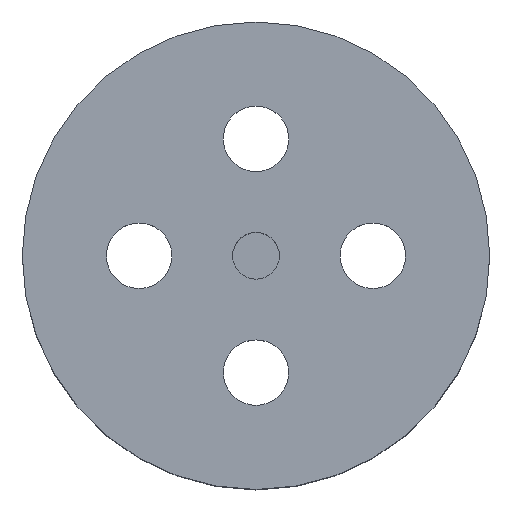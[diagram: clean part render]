
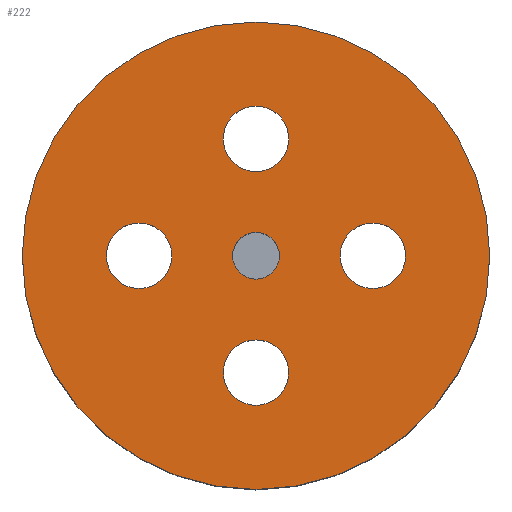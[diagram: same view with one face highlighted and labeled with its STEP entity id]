
A CAD part, top view. The second image highlights one B-rep face of the part: STEP entity #222.
In plain terms, the highlighted planar face has unit normal (0, 0, 1).
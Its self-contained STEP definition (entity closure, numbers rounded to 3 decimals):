
#18 = ORIENTED_EDGE ( 'NONE', *, *, #85, .F. ) ;
#62 = EDGE_CURVE ( 'NONE', #857, #853, #886, .T. ) ;
#64 = EDGE_CURVE ( 'NONE', #859, #860, #882, .T. ) ;
#68 = EDGE_CURVE ( 'NONE', #858, #1016, #864, .T. ) ;
#73 = EDGE_CURVE ( 'NONE', #861, #1049, #862, .T. ) ;
#85 = EDGE_CURVE ( 'NONE', #769, #775, #551, .T. ) ;
#86 = EDGE_CURVE ( 'NONE', #1076, #1083, #544, .T. ) ;
#87 = EDGE_CURVE ( 'NONE', #1049, #861, #519, .T. ) ;
#88 = EDGE_CURVE ( 'NONE', #1016, #858, #550, .T. ) ;
#89 = EDGE_CURVE ( 'NONE', #853, #857, #558, .T. ) ;
#90 = EDGE_CURVE ( 'NONE', #860, #859, #559, .T. ) ;
#101 = EDGE_CURVE ( 'NONE', #775, #769, #538, .T. ) ;
#116 = AXIS2_PLACEMENT_3D ( 'NONE', #666, #665, #660 ) ;
#117 = AXIS2_PLACEMENT_3D ( 'NONE', #662, #659, #658 ) ;
#120 = AXIS2_PLACEMENT_3D ( 'NONE', #636, #621, #619 ) ;
#122 = AXIS2_PLACEMENT_3D ( 'NONE', #591, #635, #608 ) ;
#128 = AXIS2_PLACEMENT_3D ( 'NONE', #626, #625, #598 ) ;
#129 = AXIS2_PLACEMENT_3D ( 'NONE', #642, #640, #639 ) ;
#130 = AXIS2_PLACEMENT_3D ( 'NONE', #652, #654, #628 ) ;
#131 = AXIS2_PLACEMENT_3D ( 'NONE', #651, #638, #627 ) ;
#132 = AXIS2_PLACEMENT_3D ( 'NONE', #630, #607, #606 ) ;
#133 = AXIS2_PLACEMENT_3D ( 'NONE', #1129, #1096, #1113 ) ;
#137 = AXIS2_PLACEMENT_3D ( 'NONE', #1097, #1091, #1127 ) ;
#155 = AXIS2_PLACEMENT_3D ( 'NONE', #252, #254, #255 ) ;
#184 = AXIS2_PLACEMENT_3D ( 'NONE', #392, #393, #394 ) ;
#222 = ADVANCED_FACE ( 'NONE', ( #529, #553, #557, #505, #562, #517 ), #251, .T. ) ;
#251 = PLANE ( 'NONE',  #155 ) ;
#252 = CARTESIAN_POINT ( 'NONE',  ( 0., 0., 30. ) ) ;
#254 = DIRECTION ( 'NONE',  ( 0., 0., 1. ) ) ;
#255 = DIRECTION ( 'NONE',  ( 1., 0., 0. ) ) ;
#352 = CARTESIAN_POINT ( 'NONE',  ( -3.5, 12.5, 30. ) ) ;
#357 = CARTESIAN_POINT ( 'NONE',  ( 2.5, 0., 30. ) ) ;
#358 = CARTESIAN_POINT ( 'NONE',  ( -2.5, 0., 30. ) ) ;
#364 = CARTESIAN_POINT ( 'NONE',  ( -16., 0., 30. ) ) ;
#365 = CARTESIAN_POINT ( 'NONE',  ( 3.5, -12.5, 30. ) ) ;
#367 = CARTESIAN_POINT ( 'NONE',  ( -3.5, -12.5, 30. ) ) ;
#368 = CARTESIAN_POINT ( 'NONE',  ( 9., 0., 30. ) ) ;
#369 = CARTESIAN_POINT ( 'NONE',  ( 16., 0., 30. ) ) ;
#392 = CARTESIAN_POINT ( 'NONE',  ( 0., 0., 30. ) ) ;
#393 = DIRECTION ( 'NONE',  ( 0., 0., 1. ) ) ;
#394 = DIRECTION ( 'NONE',  ( 1., 0., 0. ) ) ;
#396 = CARTESIAN_POINT ( 'NONE',  ( -9., 0., 30. ) ) ;
#422 = CARTESIAN_POINT ( 'NONE',  ( 3.5, 12.5, 30. ) ) ;
#428 = CARTESIAN_POINT ( 'NONE',  ( -25., 0., 30. ) ) ;
#440 = CARTESIAN_POINT ( 'NONE',  ( 25., 0., 30. ) ) ;
#505 = FACE_BOUND ( 'NONE', #1166, .T. ) ;
#517 = FACE_BOUND ( 'NONE', #1155, .T. ) ;
#519 = CIRCLE ( 'NONE', #130, 3.5 ) ;
#529 = FACE_BOUND ( 'NONE', #1050, .T. ) ;
#538 = CIRCLE ( 'NONE', #137, 2.5 ) ;
#544 = CIRCLE ( 'NONE', #129, 25. ) ;
#550 = CIRCLE ( 'NONE', #131, 3.5 ) ;
#551 = CIRCLE ( 'NONE', #128, 2.5 ) ;
#553 = FACE_BOUND ( 'NONE', #1216, .T. ) ;
#557 = FACE_BOUND ( 'NONE', #1028, .T. ) ;
#558 = CIRCLE ( 'NONE', #132, 3.5 ) ;
#559 = CIRCLE ( 'NONE', #133, 3.5 ) ;
#562 = FACE_OUTER_BOUND ( 'NONE', #1225, .T. ) ;
#591 = CARTESIAN_POINT ( 'NONE',  ( 0., 12.5, 30. ) ) ;
#598 = DIRECTION ( 'NONE',  ( 1., 0., 0. ) ) ;
#606 = DIRECTION ( 'NONE',  ( 1., 0., 0. ) ) ;
#607 = DIRECTION ( 'NONE',  ( 0., 0., 1. ) ) ;
#608 = DIRECTION ( 'NONE',  ( 1., 0., 0. ) ) ;
#619 = DIRECTION ( 'NONE',  ( 1., 0., 0. ) ) ;
#621 = DIRECTION ( 'NONE',  ( 0., 0., 1. ) ) ;
#625 = DIRECTION ( 'NONE',  ( 0., 0., 1. ) ) ;
#626 = CARTESIAN_POINT ( 'NONE',  ( 0., 0., 30. ) ) ;
#627 = DIRECTION ( 'NONE',  ( 1., 0., 0. ) ) ;
#628 = DIRECTION ( 'NONE',  ( 1., 0., 0. ) ) ;
#630 = CARTESIAN_POINT ( 'NONE',  ( 0., -12.5, 30. ) ) ;
#635 = DIRECTION ( 'NONE',  ( 0., 0., 1. ) ) ;
#636 = CARTESIAN_POINT ( 'NONE',  ( -12.5, 0., 30. ) ) ;
#638 = DIRECTION ( 'NONE',  ( 0., 0., 1. ) ) ;
#639 = DIRECTION ( 'NONE',  ( 1., 0., 0. ) ) ;
#640 = DIRECTION ( 'NONE',  ( 0., 0., 1. ) ) ;
#642 = CARTESIAN_POINT ( 'NONE',  ( 0., 0., 30. ) ) ;
#651 = CARTESIAN_POINT ( 'NONE',  ( -12.5, 0., 30. ) ) ;
#652 = CARTESIAN_POINT ( 'NONE',  ( 0., 12.5, 30. ) ) ;
#654 = DIRECTION ( 'NONE',  ( 0., 0., 1. ) ) ;
#658 = DIRECTION ( 'NONE',  ( 1., 0., 0. ) ) ;
#659 = DIRECTION ( 'NONE',  ( 0., 0., 1. ) ) ;
#660 = DIRECTION ( 'NONE',  ( 1., 0., 0. ) ) ;
#662 = CARTESIAN_POINT ( 'NONE',  ( 12.5, 0., 30. ) ) ;
#665 = DIRECTION ( 'NONE',  ( 0., 0., 1. ) ) ;
#666 = CARTESIAN_POINT ( 'NONE',  ( 0., -12.5, 30. ) ) ;
#769 = VERTEX_POINT ( 'NONE', #357 ) ;
#775 = VERTEX_POINT ( 'NONE', #358 ) ;
#853 = VERTEX_POINT ( 'NONE', #365 ) ;
#857 = VERTEX_POINT ( 'NONE', #367 ) ;
#858 = VERTEX_POINT ( 'NONE', #364 ) ;
#859 = VERTEX_POINT ( 'NONE', #368 ) ;
#860 = VERTEX_POINT ( 'NONE', #369 ) ;
#861 = VERTEX_POINT ( 'NONE', #352 ) ;
#862 = CIRCLE ( 'NONE', #122, 3.5 ) ;
#864 = CIRCLE ( 'NONE', #120, 3.5 ) ;
#882 = CIRCLE ( 'NONE', #117, 3.5 ) ;
#886 = CIRCLE ( 'NONE', #116, 3.5 ) ;
#949 = EDGE_CURVE ( 'NONE', #1083, #1076, #973, .T. ) ;
#973 = CIRCLE ( 'NONE', #184, 25. ) ;
#1016 = VERTEX_POINT ( 'NONE', #396 ) ;
#1028 = EDGE_LOOP ( 'NONE', ( #1148, #1264 ) ) ;
#1049 = VERTEX_POINT ( 'NONE', #422 ) ;
#1050 = EDGE_LOOP ( 'NONE', ( #1145, #1275 ) ) ;
#1076 = VERTEX_POINT ( 'NONE', #428 ) ;
#1083 = VERTEX_POINT ( 'NONE', #440 ) ;
#1091 = DIRECTION ( 'NONE',  ( 0., 0., 1. ) ) ;
#1096 = DIRECTION ( 'NONE',  ( 0., 0., 1. ) ) ;
#1097 = CARTESIAN_POINT ( 'NONE',  ( 0., 0., 30. ) ) ;
#1113 = DIRECTION ( 'NONE',  ( 1., 0., 0. ) ) ;
#1127 = DIRECTION ( 'NONE',  ( 1., 0., 0. ) ) ;
#1129 = CARTESIAN_POINT ( 'NONE',  ( 12.5, 0., 30. ) ) ;
#1145 = ORIENTED_EDGE ( 'NONE', *, *, #64, .F. ) ;
#1148 = ORIENTED_EDGE ( 'NONE', *, *, #68, .F. ) ;
#1155 = EDGE_LOOP ( 'NONE', ( #18, #1215 ) ) ;
#1166 = EDGE_LOOP ( 'NONE', ( #1222, #1223 ) ) ;
#1213 = ORIENTED_EDGE ( 'NONE', *, *, #86, .T. ) ;
#1215 = ORIENTED_EDGE ( 'NONE', *, *, #101, .F. ) ;
#1216 = EDGE_LOOP ( 'NONE', ( #1220, #1266 ) ) ;
#1220 = ORIENTED_EDGE ( 'NONE', *, *, #62, .F. ) ;
#1222 = ORIENTED_EDGE ( 'NONE', *, *, #73, .F. ) ;
#1223 = ORIENTED_EDGE ( 'NONE', *, *, #87, .F. ) ;
#1225 = EDGE_LOOP ( 'NONE', ( #1213, #1248 ) ) ;
#1248 = ORIENTED_EDGE ( 'NONE', *, *, #949, .T. ) ;
#1264 = ORIENTED_EDGE ( 'NONE', *, *, #88, .F. ) ;
#1266 = ORIENTED_EDGE ( 'NONE', *, *, #89, .F. ) ;
#1275 = ORIENTED_EDGE ( 'NONE', *, *, #90, .F. ) ;
